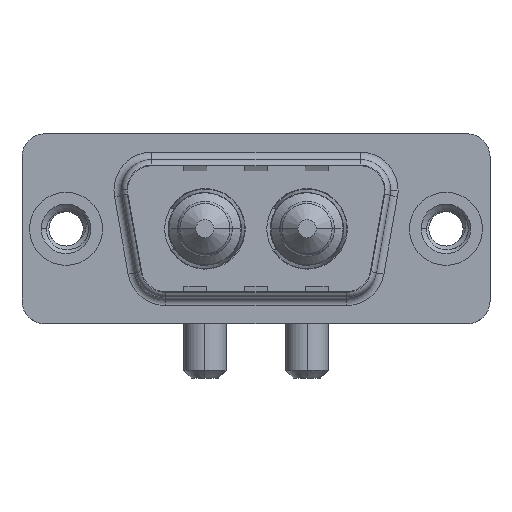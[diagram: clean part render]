
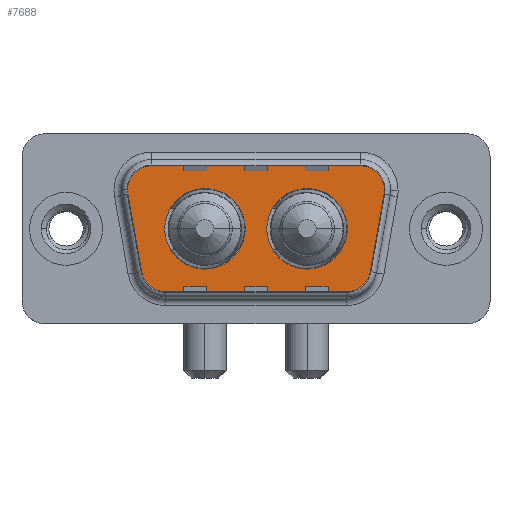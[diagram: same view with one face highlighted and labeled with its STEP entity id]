
A CAD part, top view. The second image highlights one B-rep face of the part: STEP entity #7688.
In plain terms, the highlighted planar face has unit normal (0, 0, 1).
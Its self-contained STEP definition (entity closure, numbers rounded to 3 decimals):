
#38 = EDGE_CURVE ( 'NONE', #2544, #4970, #134, .T. ) ;
#79 = CARTESIAN_POINT ( 'NONE',  ( 19.564, 2.9, 0. ) ) ;
#134 = LINE ( 'NONE', #8064, #8195 ) ;
#238 = PLANE ( 'NONE',  #2058 ) ;
#291 = ORIENTED_EDGE ( 'NONE', *, *, #3452, .F. ) ;
#347 = FACE_BOUND ( 'NONE', #7420, .T. ) ;
#896 = ORIENTED_EDGE ( 'NONE', *, *, #5592, .T. ) ;
#898 = CARTESIAN_POINT ( 'NONE',  ( 3.466, 2.553, 0. ) ) ;
#1082 = CARTESIAN_POINT ( 'NONE',  ( 9.14, 0., 0. ) ) ;
#1130 = VECTOR ( 'NONE', #11275, 1000. ) ;
#1235 = CARTESIAN_POINT ( 'NONE',  ( 18.51, 0., 0. ) ) ;
#1488 = CIRCLE ( 'NONE', #8048, 2.65 ) ;
#1502 = CARTESIAN_POINT ( 'NONE',  ( 5.436, 2.9, 0. ) ) ;
#1624 = DIRECTION ( 'NONE',  ( 1., 0., 0. ) ) ;
#1665 = AXIS2_PLACEMENT_3D ( 'NONE', #79, #2712, #7346 ) ;
#2038 = CARTESIAN_POINT ( 'NONE',  ( 13.21, 0., 0. ) ) ;
#2058 = AXIS2_PLACEMENT_3D ( 'NONE', #9441, #5735, #2110 ) ;
#2099 = VERTEX_POINT ( 'NONE', #5253 ) ;
#2110 = DIRECTION ( 'NONE',  ( 1., 0., 0. ) ) ;
#2296 = VERTEX_POINT ( 'NONE', #2615 ) ;
#2306 = EDGE_CURVE ( 'NONE', #9693, #9666, #9889, .T. ) ;
#2355 = DIRECTION ( 'NONE',  ( 0., 0., 1. ) ) ;
#2402 = ORIENTED_EDGE ( 'NONE', *, *, #8966, .T. ) ;
#2544 = VERTEX_POINT ( 'NONE', #7170 ) ;
#2615 = CARTESIAN_POINT ( 'NONE',  ( 6.49, 0., 0. ) ) ;
#2617 = CARTESIAN_POINT ( 'NONE',  ( 4.489, -3.247, 0. ) ) ;
#2642 = LINE ( 'NONE', #898, #7851 ) ;
#2712 = DIRECTION ( 'NONE',  ( 0., 0., 1. ) ) ;
#2781 = CIRCLE ( 'NONE', #9341, 2.65 ) ;
#2813 = CIRCLE ( 'NONE', #4313, 2. ) ;
#2928 = DIRECTION ( 'NONE',  ( 0., 0., 1. ) ) ;
#3167 = EDGE_CURVE ( 'NONE', #4970, #10233, #4740, .T. ) ;
#3227 = DIRECTION ( 'NONE',  ( 1., 0., 0. ) ) ;
#3234 = CARTESIAN_POINT ( 'NONE',  ( 6.459, -2.9, 0. ) ) ;
#3452 = EDGE_CURVE ( 'NONE', #4012, #11216, #6281, .T. ) ;
#3764 = CARTESIAN_POINT ( 'NONE',  ( 15.86, 0., 0. ) ) ;
#4009 = CARTESIAN_POINT ( 'NONE',  ( 15.86, 0., 0. ) ) ;
#4012 = VERTEX_POINT ( 'NONE', #1235 ) ;
#4015 = EDGE_CURVE ( 'NONE', #5880, #2296, #6347, .T. ) ;
#4151 = CARTESIAN_POINT ( 'NONE',  ( 5.436, 4.9, 0. ) ) ;
#4313 = AXIS2_PLACEMENT_3D ( 'NONE', #10343, #2928, #10103 ) ;
#4372 = EDGE_CURVE ( 'NONE', #11216, #4012, #1488, .T. ) ;
#4673 = EDGE_LOOP ( 'NONE', ( #291, #9071 ) ) ;
#4740 = CIRCLE ( 'NONE', #9643, 2. ) ;
#4840 = CARTESIAN_POINT ( 'NONE',  ( 6.459, -4.9, 0. ) ) ;
#4970 = VERTEX_POINT ( 'NONE', #8637 ) ;
#5176 = ORIENTED_EDGE ( 'NONE', *, *, #5916, .F. ) ;
#5253 = CARTESIAN_POINT ( 'NONE',  ( 19.564, 4.9, 0. ) ) ;
#5378 = CARTESIAN_POINT ( 'NONE',  ( 3.466, 2.553, 0. ) ) ;
#5564 = CIRCLE ( 'NONE', #1665, 2. ) ;
#5592 = EDGE_CURVE ( 'NONE', #7899, #10531, #6089, .T. ) ;
#5718 = DIRECTION ( 'NONE',  ( 0., 0., 1. ) ) ;
#5735 = DIRECTION ( 'NONE',  ( 0., 0., 1. ) ) ;
#5789 = CARTESIAN_POINT ( 'NONE',  ( 21.564, 2.9, 0. ) ) ;
#5870 = LINE ( 'NONE', #9502, #1130 ) ;
#5880 = VERTEX_POINT ( 'NONE', #11043 ) ;
#5916 = EDGE_CURVE ( 'NONE', #2296, #5880, #2781, .T. ) ;
#5956 = EDGE_LOOP ( 'NONE', ( #7666, #9060, #11546, #2402, #8815, #896, #11143, #8079, #10516 ) ) ;
#6002 = CIRCLE ( 'NONE', #10866, 2. ) ;
#6089 = CIRCLE ( 'NONE', #8507, 2. ) ;
#6196 = CARTESIAN_POINT ( 'NONE',  ( 6.459, -4.9, 0. ) ) ;
#6281 = CIRCLE ( 'NONE', #10209, 2.65 ) ;
#6347 = CIRCLE ( 'NONE', #7662, 2.65 ) ;
#6523 = DIRECTION ( 'NONE',  ( 0., 0., 1. ) ) ;
#6566 = FACE_OUTER_BOUND ( 'NONE', #5956, .T. ) ;
#6903 = CARTESIAN_POINT ( 'NONE',  ( 19.564, 2.9, 0. ) ) ;
#6998 = VECTOR ( 'NONE', #9952, 1000. ) ;
#7057 = EDGE_CURVE ( 'NONE', #2099, #7899, #5870, .T. ) ;
#7143 = EDGE_CURVE ( 'NONE', #11544, #9693, #6002, .T. ) ;
#7170 = CARTESIAN_POINT ( 'NONE',  ( 20.511, -3.247, 0. ) ) ;
#7323 = EDGE_CURVE ( 'NONE', #9666, #2544, #2813, .T. ) ;
#7346 = DIRECTION ( 'NONE',  ( -1., 0., 0. ) ) ;
#7371 = DIRECTION ( 'NONE',  ( 0., 0., 1. ) ) ;
#7420 = EDGE_LOOP ( 'NONE', ( #8721, #5176 ) ) ;
#7497 = CARTESIAN_POINT ( 'NONE',  ( 18.541, -4.9, 0. ) ) ;
#7514 = DIRECTION ( 'NONE',  ( 0., 0., 1. ) ) ;
#7662 = AXIS2_PLACEMENT_3D ( 'NONE', #8384, #7514, #3227 ) ;
#7666 = ORIENTED_EDGE ( 'NONE', *, *, #7323, .T. ) ;
#7688 = ADVANCED_FACE ( 'NONE', ( #10965, #347, #6566 ), #238, .T. ) ;
#7851 = VECTOR ( 'NONE', #10027, 1000. ) ;
#7899 = VERTEX_POINT ( 'NONE', #4151 ) ;
#8048 = AXIS2_PLACEMENT_3D ( 'NONE', #4009, #5718, #10246 ) ;
#8064 = CARTESIAN_POINT ( 'NONE',  ( 21.534, 2.553, 0. ) ) ;
#8079 = ORIENTED_EDGE ( 'NONE', *, *, #7143, .T. ) ;
#8195 = VECTOR ( 'NONE', #9878, 1000. ) ;
#8283 = DIRECTION ( 'NONE',  ( 1., 0., 0. ) ) ;
#8384 = CARTESIAN_POINT ( 'NONE',  ( 9.14, 0., 0. ) ) ;
#8507 = AXIS2_PLACEMENT_3D ( 'NONE', #1502, #11355, #1624 ) ;
#8637 = CARTESIAN_POINT ( 'NONE',  ( 21.534, 2.553, 0. ) ) ;
#8721 = ORIENTED_EDGE ( 'NONE', *, *, #4015, .F. ) ;
#8815 = ORIENTED_EDGE ( 'NONE', *, *, #7057, .T. ) ;
#8841 = DIRECTION ( 'NONE',  ( -1., 0., 0. ) ) ;
#8966 = EDGE_CURVE ( 'NONE', #10233, #2099, #5564, .T. ) ;
#9060 = ORIENTED_EDGE ( 'NONE', *, *, #38, .T. ) ;
#9071 = ORIENTED_EDGE ( 'NONE', *, *, #4372, .F. ) ;
#9341 = AXIS2_PLACEMENT_3D ( 'NONE', #1082, #6523, #8283 ) ;
#9441 = CARTESIAN_POINT ( 'NONE',  ( 18.541, -2.9, 0. ) ) ;
#9502 = CARTESIAN_POINT ( 'NONE',  ( 5.436, 4.9, 0. ) ) ;
#9554 = EDGE_CURVE ( 'NONE', #10531, #11544, #2642, .T. ) ;
#9643 = AXIS2_PLACEMENT_3D ( 'NONE', #6903, #9667, #8841 ) ;
#9666 = VERTEX_POINT ( 'NONE', #7497 ) ;
#9667 = DIRECTION ( 'NONE',  ( 0., 0., 1. ) ) ;
#9693 = VERTEX_POINT ( 'NONE', #4840 ) ;
#9820 = DIRECTION ( 'NONE',  ( -1., 0., 0. ) ) ;
#9878 = DIRECTION ( 'NONE',  ( 0.174, 0.985, 0. ) ) ;
#9889 = LINE ( 'NONE', #6196, #6998 ) ;
#9952 = DIRECTION ( 'NONE',  ( 1., 0., 0. ) ) ;
#10027 = DIRECTION ( 'NONE',  ( 0.174, -0.985, 0. ) ) ;
#10103 = DIRECTION ( 'NONE',  ( 1., 0., 0. ) ) ;
#10209 = AXIS2_PLACEMENT_3D ( 'NONE', #3764, #7371, #10938 ) ;
#10233 = VERTEX_POINT ( 'NONE', #5789 ) ;
#10246 = DIRECTION ( 'NONE',  ( 1., 0., 0. ) ) ;
#10343 = CARTESIAN_POINT ( 'NONE',  ( 18.541, -2.9, 0. ) ) ;
#10516 = ORIENTED_EDGE ( 'NONE', *, *, #2306, .T. ) ;
#10531 = VERTEX_POINT ( 'NONE', #5378 ) ;
#10866 = AXIS2_PLACEMENT_3D ( 'NONE', #3234, #2355, #9820 ) ;
#10938 = DIRECTION ( 'NONE',  ( 1., 0., 0. ) ) ;
#10965 = FACE_BOUND ( 'NONE', #4673, .T. ) ;
#11043 = CARTESIAN_POINT ( 'NONE',  ( 11.79, 0., 0. ) ) ;
#11143 = ORIENTED_EDGE ( 'NONE', *, *, #9554, .T. ) ;
#11216 = VERTEX_POINT ( 'NONE', #2038 ) ;
#11275 = DIRECTION ( 'NONE',  ( -1., 0., 0. ) ) ;
#11355 = DIRECTION ( 'NONE',  ( 0., 0., 1. ) ) ;
#11544 = VERTEX_POINT ( 'NONE', #2617 ) ;
#11546 = ORIENTED_EDGE ( 'NONE', *, *, #3167, .T. ) ;
